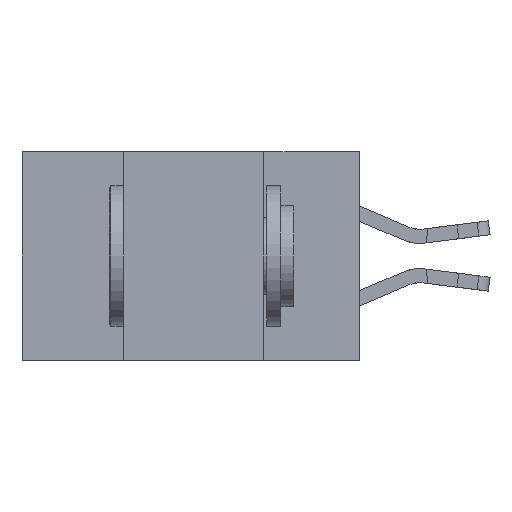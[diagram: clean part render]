
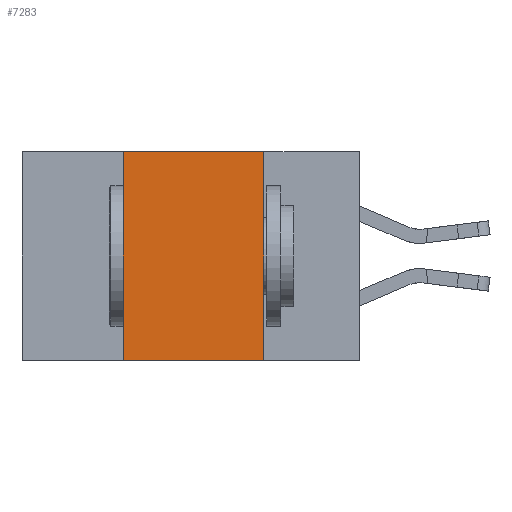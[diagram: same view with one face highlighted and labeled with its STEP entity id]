
A CAD part, left-side view. The second image highlights one B-rep face of the part: STEP entity #7283.
In plain terms, the highlighted planar face has unit normal (-1, 0, 0).
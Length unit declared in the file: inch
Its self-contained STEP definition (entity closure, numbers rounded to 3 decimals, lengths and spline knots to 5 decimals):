
#508 = VERTEX_POINT ( 'NONE', #17572 ) ;
#911 = LINE ( 'NONE', #2858, #10181 ) ;
#1020 = EDGE_LOOP ( 'NONE', ( #6281, #7288, #13601, #19002 ) ) ;
#2590 = CARTESIAN_POINT ( 'NONE',  ( 0., 0.6, -0.37 ) ) ;
#2653 = DIRECTION ( 'NONE',  ( 0., -1., 0. ) ) ;
#2858 = CARTESIAN_POINT ( 'NONE',  ( 0., 0.42, 0. ) ) ;
#2925 = DIRECTION ( 'NONE',  ( 0., 0., 1. ) ) ;
#3208 = EDGE_CURVE ( 'NONE', #12047, #12553, #15137, .T. ) ;
#3664 = DIRECTION ( 'NONE',  ( 1., 0., 0. ) ) ;
#4303 = EDGE_CURVE ( 'NONE', #9569, #12553, #12361, .T. ) ;
#5698 = VECTOR ( 'NONE', #18682, 39.37008 ) ;
#6281 = ORIENTED_EDGE ( 'NONE', *, *, #3208, .F. ) ;
#6469 = AXIS2_PLACEMENT_3D ( 'NONE', #16988, #3664, #12682 ) ;
#7283 = ADVANCED_FACE ( 'NONE', ( #17715 ), #12638, .F. ) ;
#7288 = ORIENTED_EDGE ( 'NONE', *, *, #16531, .F. ) ;
#9569 = VERTEX_POINT ( 'NONE', #10180 ) ;
#10180 = CARTESIAN_POINT ( 'NONE',  ( 0., 0.42, -0.37 ) ) ;
#10181 = VECTOR ( 'NONE', #2925, 39.37008 ) ;
#11319 = CARTESIAN_POINT ( 'NONE',  ( 0., 0.17, 0. ) ) ;
#12047 = VERTEX_POINT ( 'NONE', #17620 ) ;
#12264 = CARTESIAN_POINT ( 'NONE',  ( 0., 0.17, -0.37 ) ) ;
#12361 = LINE ( 'NONE', #2590, #17195 ) ;
#12553 = VERTEX_POINT ( 'NONE', #12264 ) ;
#12638 = PLANE ( 'NONE',  #6469 ) ;
#12682 = DIRECTION ( 'NONE',  ( 0., 0., -1. ) ) ;
#13177 = DIRECTION ( 'NONE',  ( 0., -1., 0. ) ) ;
#13601 = ORIENTED_EDGE ( 'NONE', *, *, #14564, .F. ) ;
#13960 = VECTOR ( 'NONE', #13177, 39.37008 ) ;
#14564 = EDGE_CURVE ( 'NONE', #9569, #508, #911, .T. ) ;
#15137 = LINE ( 'NONE', #11319, #5698 ) ;
#16531 = EDGE_CURVE ( 'NONE', #508, #12047, #18369, .T. ) ;
#16988 = CARTESIAN_POINT ( 'NONE',  ( 0., 0.6, 0. ) ) ;
#17195 = VECTOR ( 'NONE', #2653, 39.37008 ) ;
#17572 = CARTESIAN_POINT ( 'NONE',  ( 0., 0.42, 0. ) ) ;
#17620 = CARTESIAN_POINT ( 'NONE',  ( 0., 0.17, 0. ) ) ;
#17682 = CARTESIAN_POINT ( 'NONE',  ( 0., 0.6, 0. ) ) ;
#17715 = FACE_OUTER_BOUND ( 'NONE', #1020, .T. ) ;
#18369 = LINE ( 'NONE', #17682, #13960 ) ;
#18682 = DIRECTION ( 'NONE',  ( 0., 0., -1. ) ) ;
#19002 = ORIENTED_EDGE ( 'NONE', *, *, #4303, .T. ) ;
